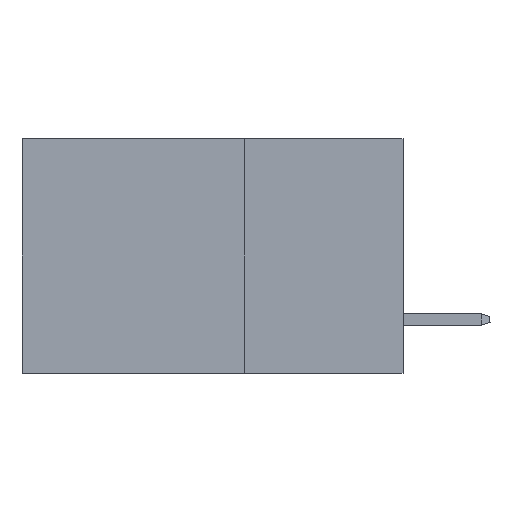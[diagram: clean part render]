
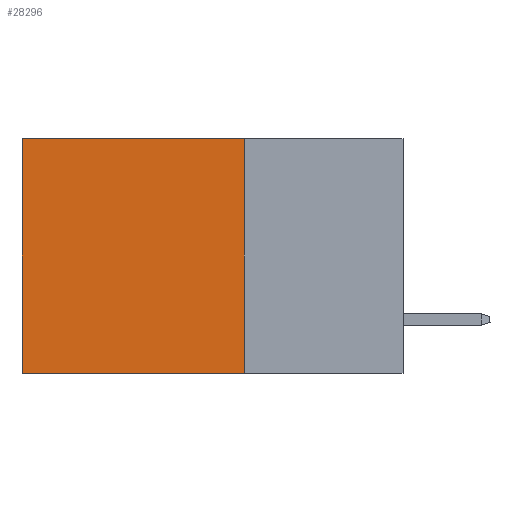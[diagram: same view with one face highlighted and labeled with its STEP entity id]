
A CAD part, left-side view. The second image highlights one B-rep face of the part: STEP entity #28296.
In plain terms, the highlighted planar face has unit normal (-1, 0, 0).
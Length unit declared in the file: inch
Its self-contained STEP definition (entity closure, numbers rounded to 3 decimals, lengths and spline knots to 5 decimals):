
#572 = VECTOR ( 'NONE', #5691, 39.37008 ) ;
#1029 = PLANE ( 'NONE',  #21826 ) ;
#1081 = LINE ( 'NONE', #4319, #1946 ) ;
#1761 = DIRECTION ( 'NONE',  ( 0., 1., 0. ) ) ;
#1946 = VECTOR ( 'NONE', #1761, 39.37008 ) ;
#2054 = CARTESIAN_POINT ( 'NONE',  ( 0.2875, 0.25, 0. ) ) ;
#2396 = LINE ( 'NONE', #2054, #4411 ) ;
#3253 = DIRECTION ( 'NONE',  ( 0., 0., -1. ) ) ;
#3460 = ORIENTED_EDGE ( 'NONE', *, *, #24141, .T. ) ;
#4319 = CARTESIAN_POINT ( 'NONE',  ( 0.2875, 0.25, 0. ) ) ;
#4411 = VECTOR ( 'NONE', #22760, 39.37008 ) ;
#5691 = DIRECTION ( 'NONE',  ( 0., 0., -1. ) ) ;
#6066 = VECTOR ( 'NONE', #32079, 39.37008 ) ;
#7123 = CARTESIAN_POINT ( 'NONE',  ( 0.2875, 0.25, 0. ) ) ;
#8359 = DIRECTION ( 'NONE',  ( 1., 0., 0. ) ) ;
#9877 = EDGE_CURVE ( 'NONE', #10925, #24523, #1081, .T. ) ;
#10851 = CARTESIAN_POINT ( 'NONE',  ( 0.2875, 0.6, -0.37 ) ) ;
#10925 = VERTEX_POINT ( 'NONE', #7123 ) ;
#13297 = CARTESIAN_POINT ( 'NONE',  ( 0.2875, 0.6, 0. ) ) ;
#16164 = FACE_OUTER_BOUND ( 'NONE', #31549, .T. ) ;
#20857 = VERTEX_POINT ( 'NONE', #10851 ) ;
#21133 = LINE ( 'NONE', #31814, #572 ) ;
#21241 = CARTESIAN_POINT ( 'NONE',  ( 0.2875, 0.25, 0. ) ) ;
#21826 = AXIS2_PLACEMENT_3D ( 'NONE', #21241, #8359, #3253 ) ;
#22760 = DIRECTION ( 'NONE',  ( 0., 0., -1. ) ) ;
#23074 = ORIENTED_EDGE ( 'NONE', *, *, #27060, .F. ) ;
#23610 = CARTESIAN_POINT ( 'NONE',  ( 0.2875, 0.25, -0.37 ) ) ;
#23613 = ORIENTED_EDGE ( 'NONE', *, *, #9877, .T. ) ;
#23953 = LINE ( 'NONE', #23610, #6066 ) ;
#24141 = EDGE_CURVE ( 'NONE', #24523, #20857, #21133, .T. ) ;
#24523 = VERTEX_POINT ( 'NONE', #13297 ) ;
#24878 = EDGE_CURVE ( 'NONE', #10925, #33196, #2396, .T. ) ;
#27060 = EDGE_CURVE ( 'NONE', #33196, #20857, #23953, .T. ) ;
#28296 = ADVANCED_FACE ( 'NONE', ( #16164 ), #1029, .F. ) ;
#30010 = CARTESIAN_POINT ( 'NONE',  ( 0.2875, 0.25, -0.37 ) ) ;
#31549 = EDGE_LOOP ( 'NONE', ( #3460, #23074, #32286, #23613 ) ) ;
#31814 = CARTESIAN_POINT ( 'NONE',  ( 0.2875, 0.6, 0. ) ) ;
#32079 = DIRECTION ( 'NONE',  ( 0., 1., 0. ) ) ;
#32286 = ORIENTED_EDGE ( 'NONE', *, *, #24878, .F. ) ;
#33196 = VERTEX_POINT ( 'NONE', #30010 ) ;
